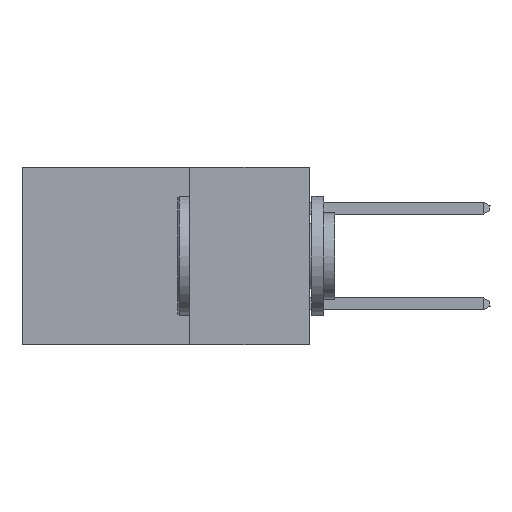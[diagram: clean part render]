
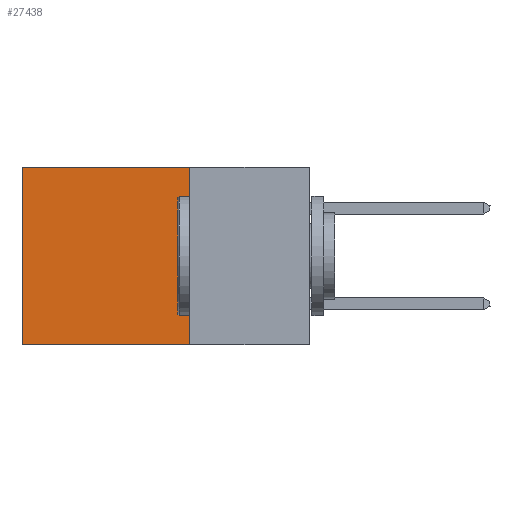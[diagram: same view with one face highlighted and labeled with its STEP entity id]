
A CAD part, left-side view. The second image highlights one B-rep face of the part: STEP entity #27438.
In plain terms, the highlighted planar face has unit normal (-1, 0, 0).
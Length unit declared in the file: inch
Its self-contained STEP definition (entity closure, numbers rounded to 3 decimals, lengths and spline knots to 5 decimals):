
#1541 = AXIS2_PLACEMENT_3D ( 'NONE', #9101, #33582, #12617 ) ;
#1980 = PLANE ( 'NONE',  #1541 ) ;
#4199 = VECTOR ( 'NONE', #25833, 39.37008 ) ;
#4312 = CARTESIAN_POINT ( 'NONE',  ( 0.2875, 0.6, -0.37 ) ) ;
#5184 = VECTOR ( 'NONE', #20084, 39.37008 ) ;
#6179 = ORIENTED_EDGE ( 'NONE', *, *, #26619, .T. ) ;
#7007 = CARTESIAN_POINT ( 'NONE',  ( 0.2875, 0.25, -0.37 ) ) ;
#9101 = CARTESIAN_POINT ( 'NONE',  ( 0.2875, 0.25, 0. ) ) ;
#11771 = CARTESIAN_POINT ( 'NONE',  ( 0.2875, 0.6, 0. ) ) ;
#12617 = DIRECTION ( 'NONE',  ( 0., 0., -1. ) ) ;
#13402 = VERTEX_POINT ( 'NONE', #37512 ) ;
#14660 = CARTESIAN_POINT ( 'NONE',  ( 0.2875, 0.6, 0. ) ) ;
#17076 = ORIENTED_EDGE ( 'NONE', *, *, #37860, .T. ) ;
#17089 = VERTEX_POINT ( 'NONE', #42898 ) ;
#17457 = VERTEX_POINT ( 'NONE', #14660 ) ;
#20084 = DIRECTION ( 'NONE',  ( 0., 0., -1. ) ) ;
#21379 = CARTESIAN_POINT ( 'NONE',  ( 0.2875, 0.25, 0. ) ) ;
#23609 = CARTESIAN_POINT ( 'NONE',  ( 0.2875, 0.25, 0. ) ) ;
#24908 = DIRECTION ( 'NONE',  ( 0., 1., 0. ) ) ;
#25833 = DIRECTION ( 'NONE',  ( 0., 0., -1. ) ) ;
#26057 = FACE_OUTER_BOUND ( 'NONE', #28767, .T. ) ;
#26619 = EDGE_CURVE ( 'NONE', #17457, #38616, #32166, .T. ) ;
#27438 = ADVANCED_FACE ( 'NONE', ( #26057 ), #1980, .F. ) ;
#28767 = EDGE_LOOP ( 'NONE', ( #6179, #33119, #29085, #17076 ) ) ;
#29085 = ORIENTED_EDGE ( 'NONE', *, *, #40305, .F. ) ;
#31240 = EDGE_CURVE ( 'NONE', #13402, #38616, #42175, .T. ) ;
#31789 = VECTOR ( 'NONE', #35031, 39.37008 ) ;
#32166 = LINE ( 'NONE', #11771, #4199 ) ;
#33119 = ORIENTED_EDGE ( 'NONE', *, *, #31240, .F. ) ;
#33582 = DIRECTION ( 'NONE',  ( 1., 0., 0. ) ) ;
#35031 = DIRECTION ( 'NONE',  ( 0., 1., 0. ) ) ;
#37512 = CARTESIAN_POINT ( 'NONE',  ( 0.2875, 0.25, -0.37 ) ) ;
#37860 = EDGE_CURVE ( 'NONE', #17089, #17457, #38188, .T. ) ;
#38188 = LINE ( 'NONE', #21379, #39292 ) ;
#38616 = VERTEX_POINT ( 'NONE', #4312 ) ;
#39292 = VECTOR ( 'NONE', #24908, 39.37008 ) ;
#40227 = LINE ( 'NONE', #23609, #5184 ) ;
#40305 = EDGE_CURVE ( 'NONE', #17089, #13402, #40227, .T. ) ;
#42175 = LINE ( 'NONE', #7007, #31789 ) ;
#42898 = CARTESIAN_POINT ( 'NONE',  ( 0.2875, 0.25, 0. ) ) ;
